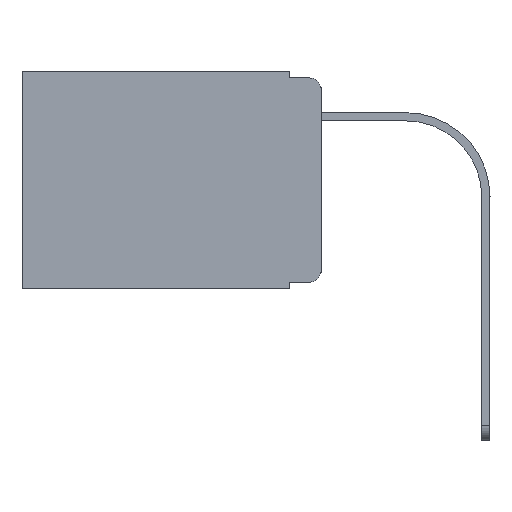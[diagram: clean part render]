
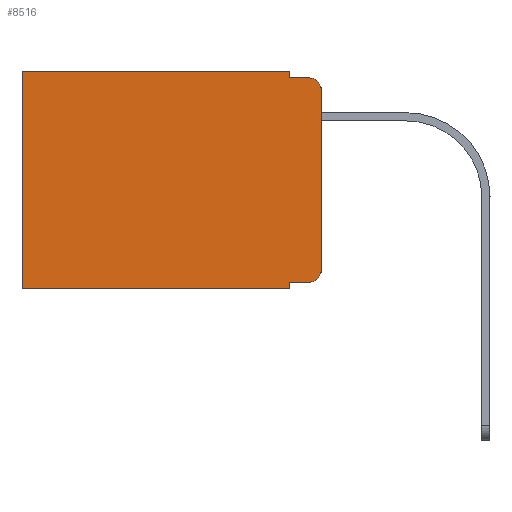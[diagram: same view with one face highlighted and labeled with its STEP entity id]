
A CAD part, left-side view. The second image highlights one B-rep face of the part: STEP entity #8516.
In plain terms, the highlighted planar face has unit normal (-1, 0, 0).
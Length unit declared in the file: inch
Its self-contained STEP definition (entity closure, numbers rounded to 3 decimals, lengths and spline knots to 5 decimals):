
#108 = VECTOR ( 'NONE', #14229, 39.37008 ) ;
#332 = DIRECTION ( 'NONE',  ( 0., 1., 0. ) ) ;
#384 = LINE ( 'NONE', #13853, #15870 ) ;
#470 = ORIENTED_EDGE ( 'NONE', *, *, #971, .T. ) ;
#498 = CARTESIAN_POINT ( 'NONE',  ( 0.298, 0.02, -0.313 ) ) ;
#925 = VECTOR ( 'NONE', #12820, 39.37008 ) ;
#971 = EDGE_CURVE ( 'NONE', #15481, #13094, #13724, .T. ) ;
#980 = EDGE_CURVE ( 'NONE', #11727, #13723, #2608, .T. ) ;
#990 = EDGE_CURVE ( 'NONE', #2470, #4980, #11964, .T. ) ;
#1487 = DIRECTION ( 'NONE',  ( 0., 0., -1. ) ) ;
#1615 = CARTESIAN_POINT ( 'NONE',  ( 0.298, 0.051, -0.01 ) ) ;
#2470 = VERTEX_POINT ( 'NONE', #4996 ) ;
#2608 = LINE ( 'NONE', #7624, #4177 ) ;
#2657 = CARTESIAN_POINT ( 'NONE',  ( 0.298, 0., -0.313 ) ) ;
#2840 = ORIENTED_EDGE ( 'NONE', *, *, #6890, .F. ) ;
#2899 = CARTESIAN_POINT ( 'NONE',  ( 0.298, 0., 0. ) ) ;
#3007 = CARTESIAN_POINT ( 'NONE',  ( 0.298, 0., -0.343 ) ) ;
#3084 = DIRECTION ( 'NONE',  ( -1., 0., 0. ) ) ;
#3240 = LINE ( 'NONE', #10283, #925 ) ;
#3372 = VECTOR ( 'NONE', #15620, 39.37008 ) ;
#3477 = CARTESIAN_POINT ( 'NONE',  ( 0.298, 0.473, 0. ) ) ;
#3616 = CARTESIAN_POINT ( 'NONE',  ( 0.298, 0.051, 0. ) ) ;
#3820 = ORIENTED_EDGE ( 'NONE', *, *, #15246, .F. ) ;
#3990 = VERTEX_POINT ( 'NONE', #1615 ) ;
#4177 = VECTOR ( 'NONE', #1487, 39.37008 ) ;
#4539 = ORIENTED_EDGE ( 'NONE', *, *, #980, .F. ) ;
#4586 = EDGE_CURVE ( 'NONE', #15840, #3990, #3240, .T. ) ;
#4735 = DIRECTION ( 'NONE',  ( -1., 0., 0. ) ) ;
#4912 = AXIS2_PLACEMENT_3D ( 'NONE', #10828, #4735, #9670 ) ;
#4980 = VERTEX_POINT ( 'NONE', #2657 ) ;
#4996 = CARTESIAN_POINT ( 'NONE',  ( 0.298, 0.02, -0.333 ) ) ;
#5225 = CARTESIAN_POINT ( 'NONE',  ( 0.298, 0., -0.03 ) ) ;
#5772 = LINE ( 'NONE', #8226, #3372 ) ;
#6298 = EDGE_CURVE ( 'NONE', #15840, #15481, #9285, .T. ) ;
#6694 = ORIENTED_EDGE ( 'NONE', *, *, #13235, .T. ) ;
#6702 = VECTOR ( 'NONE', #6757, 39.37008 ) ;
#6757 = DIRECTION ( 'NONE',  ( 0., 1., 0. ) ) ;
#6890 = EDGE_CURVE ( 'NONE', #13072, #4980, #5772, .T. ) ;
#6925 = EDGE_CURVE ( 'NONE', #13072, #10621, #11659, .T. ) ;
#7624 = CARTESIAN_POINT ( 'NONE',  ( 0.298, 0.051, 0. ) ) ;
#7857 = LINE ( 'NONE', #3007, #11285 ) ;
#8050 = LINE ( 'NONE', #13015, #108 ) ;
#8226 = CARTESIAN_POINT ( 'NONE',  ( 0.298, 0., 0. ) ) ;
#8516 = ADVANCED_FACE ( 'NONE', ( #11804 ), #10818, .F. ) ;
#8651 = CARTESIAN_POINT ( 'NONE',  ( 0.298, 0.473, -0.343 ) ) ;
#8930 = ORIENTED_EDGE ( 'NONE', *, *, #9689, .F. ) ;
#9285 = LINE ( 'NONE', #2899, #6702 ) ;
#9670 = DIRECTION ( 'NONE',  ( 0., 0., -1. ) ) ;
#9689 = EDGE_CURVE ( 'NONE', #3990, #10621, #384, .T. ) ;
#9805 = DIRECTION ( 'NONE',  ( 1., 0., 0. ) ) ;
#9859 = VECTOR ( 'NONE', #13890, 39.37008 ) ;
#10283 = CARTESIAN_POINT ( 'NONE',  ( 0.298, 0.051, 0. ) ) ;
#10550 = CARTESIAN_POINT ( 'NONE',  ( 0.298, 0.051, -0.343 ) ) ;
#10621 = VERTEX_POINT ( 'NONE', #13298 ) ;
#10818 = PLANE ( 'NONE',  #14054 ) ;
#10828 = CARTESIAN_POINT ( 'NONE',  ( 0.298, 0.02, -0.03 ) ) ;
#11140 = DIRECTION ( 'NONE',  ( 0., 0., -1. ) ) ;
#11285 = VECTOR ( 'NONE', #332, 39.37008 ) ;
#11328 = ORIENTED_EDGE ( 'NONE', *, *, #6925, .T. ) ;
#11659 = CIRCLE ( 'NONE', #4912, 0.02 ) ;
#11727 = VERTEX_POINT ( 'NONE', #12690 ) ;
#11804 = FACE_OUTER_BOUND ( 'NONE', #14539, .T. ) ;
#11964 = CIRCLE ( 'NONE', #13516, 0.02 ) ;
#12641 = DIRECTION ( 'NONE',  ( 0., -1., 0. ) ) ;
#12690 = CARTESIAN_POINT ( 'NONE',  ( 0.298, 0.051, -0.333 ) ) ;
#12771 = ORIENTED_EDGE ( 'NONE', *, *, #990, .T. ) ;
#12820 = DIRECTION ( 'NONE',  ( 0., 0., -1. ) ) ;
#13015 = CARTESIAN_POINT ( 'NONE',  ( 0.298, 0.051, -0.333 ) ) ;
#13072 = VERTEX_POINT ( 'NONE', #5225 ) ;
#13094 = VERTEX_POINT ( 'NONE', #8651 ) ;
#13235 = EDGE_CURVE ( 'NONE', #11727, #2470, #8050, .T. ) ;
#13298 = CARTESIAN_POINT ( 'NONE',  ( 0.298, 0.02, -0.01 ) ) ;
#13516 = AXIS2_PLACEMENT_3D ( 'NONE', #498, #3084, #15346 ) ;
#13723 = VERTEX_POINT ( 'NONE', #10550 ) ;
#13724 = LINE ( 'NONE', #13809, #9859 ) ;
#13809 = CARTESIAN_POINT ( 'NONE',  ( 0.298, 0.473, 0. ) ) ;
#13853 = CARTESIAN_POINT ( 'NONE',  ( 0.298, 0.051, -0.01 ) ) ;
#13890 = DIRECTION ( 'NONE',  ( 0., 0., -1. ) ) ;
#13904 = ORIENTED_EDGE ( 'NONE', *, *, #4586, .F. ) ;
#14054 = AXIS2_PLACEMENT_3D ( 'NONE', #15771, #9805, #11140 ) ;
#14229 = DIRECTION ( 'NONE',  ( 0., -1., 0. ) ) ;
#14539 = EDGE_LOOP ( 'NONE', ( #2840, #11328, #8930, #13904, #14636, #470, #3820, #4539, #6694, #12771 ) ) ;
#14636 = ORIENTED_EDGE ( 'NONE', *, *, #6298, .T. ) ;
#15246 = EDGE_CURVE ( 'NONE', #13723, #13094, #7857, .T. ) ;
#15346 = DIRECTION ( 'NONE',  ( 0., 0., -1. ) ) ;
#15481 = VERTEX_POINT ( 'NONE', #3477 ) ;
#15620 = DIRECTION ( 'NONE',  ( 0., 0., -1. ) ) ;
#15771 = CARTESIAN_POINT ( 'NONE',  ( 0.298, 0., 0. ) ) ;
#15840 = VERTEX_POINT ( 'NONE', #3616 ) ;
#15870 = VECTOR ( 'NONE', #12641, 39.37008 ) ;
